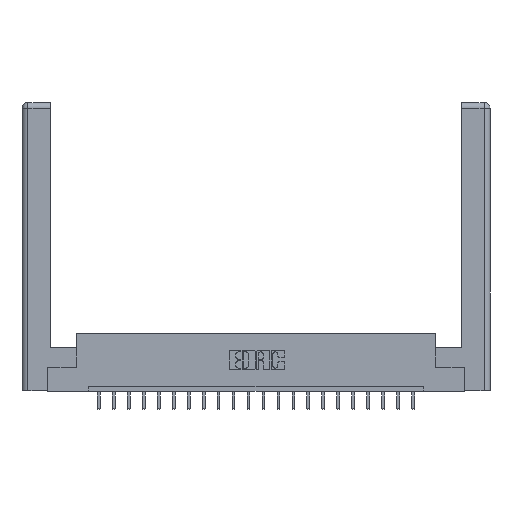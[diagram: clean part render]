
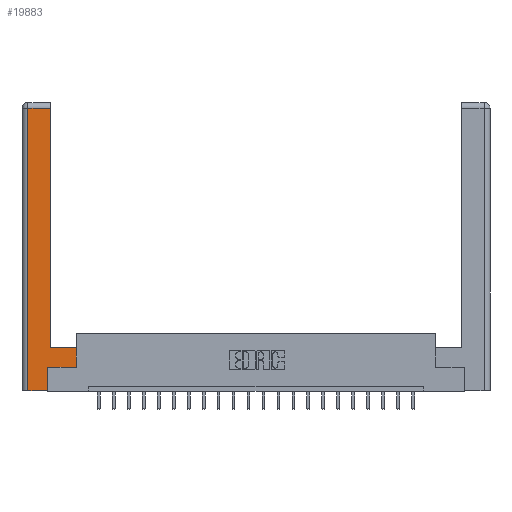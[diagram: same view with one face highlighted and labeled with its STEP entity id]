
A CAD part, top view. The second image highlights one B-rep face of the part: STEP entity #19883.
In plain terms, the highlighted planar face has unit normal (0, 0, 1).
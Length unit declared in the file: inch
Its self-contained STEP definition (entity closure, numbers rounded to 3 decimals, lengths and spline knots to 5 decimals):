
#718 = DIRECTION ( 'NONE',  ( 0., 1., 0. ) ) ;
#725 = CARTESIAN_POINT ( 'NONE',  ( 0.265, 0., 0. ) ) ;
#734 = DIRECTION ( 'NONE',  ( 0., 1., 0. ) ) ;
#1088 = EDGE_CURVE ( 'NONE', #13011, #9197, #12951, .T. ) ;
#1270 = CARTESIAN_POINT ( 'NONE',  ( 0.565, 0.245, 0. ) ) ;
#1303 = PLANE ( 'NONE',  #11233 ) ;
#1794 = CARTESIAN_POINT ( 'NONE',  ( 0.265, 0.245, 0. ) ) ;
#1820 = CARTESIAN_POINT ( 'NONE',  ( 0.265, 0.245, 0. ) ) ;
#1991 = ORIENTED_EDGE ( 'NONE', *, *, #18566, .T. ) ;
#2143 = CARTESIAN_POINT ( 'NONE',  ( 0.295, 2.94, 0. ) ) ;
#2399 = CARTESIAN_POINT ( 'NONE',  ( 0.565, 0.45, 0. ) ) ;
#2460 = CARTESIAN_POINT ( 'NONE',  ( 0.565, 0.45, 0. ) ) ;
#2749 = CARTESIAN_POINT ( 'NONE',  ( 0.565, 0.245, 0. ) ) ;
#2969 = DIRECTION ( 'NONE',  ( 0., 0., -1. ) ) ;
#3780 = EDGE_CURVE ( 'NONE', #6151, #12822, #6767, .T. ) ;
#3794 = CARTESIAN_POINT ( 'NONE',  ( 0.0615, 2.94, 0. ) ) ;
#4016 = EDGE_CURVE ( 'NONE', #7156, #19772, #4659, .T. ) ;
#4489 = DIRECTION ( 'NONE',  ( 0., -1., 0. ) ) ;
#4659 = LINE ( 'NONE', #2460, #20667 ) ;
#4727 = VERTEX_POINT ( 'NONE', #14824 ) ;
#5168 = DIRECTION ( 'NONE',  ( 1., 0., 0. ) ) ;
#5342 = DIRECTION ( 'NONE',  ( 0., 1., 0. ) ) ;
#5461 = ORIENTED_EDGE ( 'NONE', *, *, #16383, .T. ) ;
#5561 = ORIENTED_EDGE ( 'NONE', *, *, #4016, .T. ) ;
#5661 = CARTESIAN_POINT ( 'NONE',  ( 0.295, 0.45, 0. ) ) ;
#5807 = EDGE_CURVE ( 'NONE', #4727, #6151, #15606, .T. ) ;
#6151 = VERTEX_POINT ( 'NONE', #18429 ) ;
#6767 = LINE ( 'NONE', #18235, #15909 ) ;
#7062 = ORIENTED_EDGE ( 'NONE', *, *, #13778, .T. ) ;
#7156 = VERTEX_POINT ( 'NONE', #2749 ) ;
#7632 = VECTOR ( 'NONE', #5342, 39.37008 ) ;
#7807 = VECTOR ( 'NONE', #16316, 39.37008 ) ;
#8278 = VECTOR ( 'NONE', #5168, 39.37008 ) ;
#9102 = CARTESIAN_POINT ( 'NONE',  ( 0.295, 3., 0. ) ) ;
#9197 = VERTEX_POINT ( 'NONE', #2143 ) ;
#9608 = CARTESIAN_POINT ( 'NONE',  ( 0.295, 0.45, 0. ) ) ;
#10538 = ORIENTED_EDGE ( 'NONE', *, *, #1088, .T. ) ;
#11233 = AXIS2_PLACEMENT_3D ( 'NONE', #21144, #2969, #19742 ) ;
#11420 = ORIENTED_EDGE ( 'NONE', *, *, #5807, .T. ) ;
#11692 = VECTOR ( 'NONE', #734, 39.37008 ) ;
#12039 = LINE ( 'NONE', #3794, #20939 ) ;
#12198 = DIRECTION ( 'NONE',  ( -1., 0., 0. ) ) ;
#12822 = VERTEX_POINT ( 'NONE', #725 ) ;
#12951 = LINE ( 'NONE', #9102, #11692 ) ;
#13011 = VERTEX_POINT ( 'NONE', #5661 ) ;
#13355 = DIRECTION ( 'NONE',  ( 1., 0., 0. ) ) ;
#13778 = EDGE_CURVE ( 'NONE', #9197, #4727, #12039, .T. ) ;
#14359 = ORIENTED_EDGE ( 'NONE', *, *, #3780, .T. ) ;
#14393 = FACE_OUTER_BOUND ( 'NONE', #20595, .T. ) ;
#14824 = CARTESIAN_POINT ( 'NONE',  ( 0.0615, 2.94, 0. ) ) ;
#15324 = EDGE_CURVE ( 'NONE', #19772, #13011, #17270, .T. ) ;
#15606 = LINE ( 'NONE', #19516, #17984 ) ;
#15909 = VECTOR ( 'NONE', #13355, 39.37008 ) ;
#16316 = DIRECTION ( 'NONE',  ( -1., 0., 0. ) ) ;
#16383 = EDGE_CURVE ( 'NONE', #17610, #7156, #17739, .T. ) ;
#17270 = LINE ( 'NONE', #9608, #7807 ) ;
#17610 = VERTEX_POINT ( 'NONE', #1794 ) ;
#17739 = LINE ( 'NONE', #1270, #8278 ) ;
#17865 = ORIENTED_EDGE ( 'NONE', *, *, #15324, .T. ) ;
#17984 = VECTOR ( 'NONE', #4489, 39.37008 ) ;
#18235 = CARTESIAN_POINT ( 'NONE',  ( 0.265, 0., 0. ) ) ;
#18429 = CARTESIAN_POINT ( 'NONE',  ( 0.0615, 0., 0. ) ) ;
#18566 = EDGE_CURVE ( 'NONE', #12822, #17610, #19424, .T. ) ;
#19424 = LINE ( 'NONE', #1820, #7632 ) ;
#19516 = CARTESIAN_POINT ( 'NONE',  ( 0.0615, 0., 0. ) ) ;
#19742 = DIRECTION ( 'NONE',  ( -1., 0., 0. ) ) ;
#19772 = VERTEX_POINT ( 'NONE', #2399 ) ;
#19883 = ADVANCED_FACE ( 'NONE', ( #14393 ), #1303, .F. ) ;
#20595 = EDGE_LOOP ( 'NONE', ( #10538, #7062, #11420, #14359, #1991, #5461, #5561, #17865 ) ) ;
#20667 = VECTOR ( 'NONE', #718, 39.37008 ) ;
#20939 = VECTOR ( 'NONE', #12198, 39.37008 ) ;
#21144 = CARTESIAN_POINT ( 'NONE',  ( 0., 0., 0. ) ) ;
